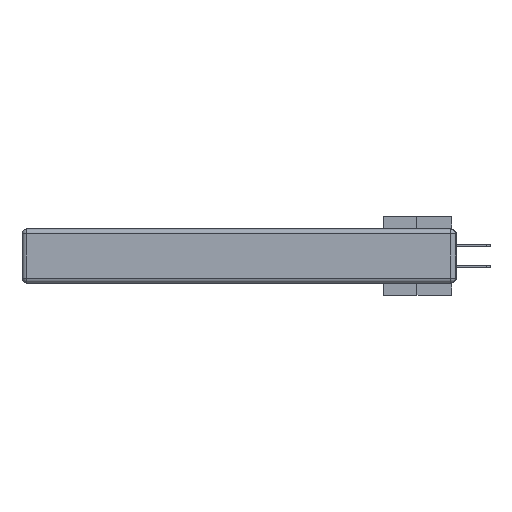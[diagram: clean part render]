
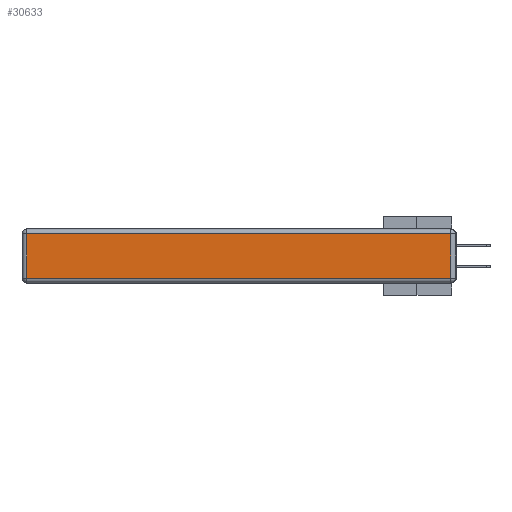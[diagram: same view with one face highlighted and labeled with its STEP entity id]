
A CAD part, left-side view. The second image highlights one B-rep face of the part: STEP entity #30633.
In plain terms, the highlighted planar face has unit normal (-1, 0, 0).
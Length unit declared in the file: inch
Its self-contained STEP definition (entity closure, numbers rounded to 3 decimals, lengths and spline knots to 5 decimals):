
#1391 = CARTESIAN_POINT ( 'NONE',  ( 0., 2.72, -0.313 ) ) ;
#1559 = EDGE_LOOP ( 'NONE', ( #24107, #34890, #33872, #4203 ) ) ;
#3076 = VERTEX_POINT ( 'NONE', #6865 ) ;
#4203 = ORIENTED_EDGE ( 'NONE', *, *, #4893, .T. ) ;
#4230 = VECTOR ( 'NONE', #23990, 39.37008 ) ;
#4887 = DIRECTION ( 'NONE',  ( 0., 1., 0. ) ) ;
#4893 = EDGE_CURVE ( 'NONE', #3076, #26150, #29987, .T. ) ;
#5307 = CARTESIAN_POINT ( 'NONE',  ( 0., 0.03, -0.03 ) ) ;
#6865 = CARTESIAN_POINT ( 'NONE',  ( 0., 2.72, -0.03 ) ) ;
#7167 = LINE ( 'NONE', #7829, #11244 ) ;
#7829 = CARTESIAN_POINT ( 'NONE',  ( 0., 2.75, -0.03 ) ) ;
#8776 = AXIS2_PLACEMENT_3D ( 'NONE', #37524, #19639, #25738 ) ;
#9156 = VERTEX_POINT ( 'NONE', #5307 ) ;
#11244 = VECTOR ( 'NONE', #4887, 39.37008 ) ;
#12343 = EDGE_CURVE ( 'NONE', #26150, #20337, #18204, .T. ) ;
#12402 = FACE_OUTER_BOUND ( 'NONE', #1559, .T. ) ;
#14143 = VECTOR ( 'NONE', #21905, 39.37008 ) ;
#14435 = PLANE ( 'NONE',  #8776 ) ;
#18204 = LINE ( 'NONE', #33095, #14143 ) ;
#19536 = DIRECTION ( 'NONE',  ( 0., 0., -1. ) ) ;
#19639 = DIRECTION ( 'NONE',  ( -1., 0., 0. ) ) ;
#20337 = VERTEX_POINT ( 'NONE', #30482 ) ;
#21905 = DIRECTION ( 'NONE',  ( 0., -1., 0. ) ) ;
#23990 = DIRECTION ( 'NONE',  ( 0., 0., 1. ) ) ;
#24107 = ORIENTED_EDGE ( 'NONE', *, *, #12343, .T. ) ;
#25439 = VECTOR ( 'NONE', #19536, 39.37008 ) ;
#25738 = DIRECTION ( 'NONE',  ( 0., 0., 1. ) ) ;
#26150 = VERTEX_POINT ( 'NONE', #1391 ) ;
#26480 = LINE ( 'NONE', #35804, #4230 ) ;
#28216 = EDGE_CURVE ( 'NONE', #9156, #3076, #7167, .T. ) ;
#29987 = LINE ( 'NONE', #36914, #25439 ) ;
#30482 = CARTESIAN_POINT ( 'NONE',  ( 0., 0.03, -0.313 ) ) ;
#30633 = ADVANCED_FACE ( 'NONE', ( #12402 ), #14435, .T. ) ;
#33095 = CARTESIAN_POINT ( 'NONE',  ( 0., 0., -0.313 ) ) ;
#33872 = ORIENTED_EDGE ( 'NONE', *, *, #28216, .T. ) ;
#34890 = ORIENTED_EDGE ( 'NONE', *, *, #36610, .T. ) ;
#35804 = CARTESIAN_POINT ( 'NONE',  ( 0., 0.03, -0.343 ) ) ;
#36610 = EDGE_CURVE ( 'NONE', #20337, #9156, #26480, .T. ) ;
#36914 = CARTESIAN_POINT ( 'NONE',  ( 0., 2.72, -0.343 ) ) ;
#37524 = CARTESIAN_POINT ( 'NONE',  ( 0., 0., -0.343 ) ) ;
